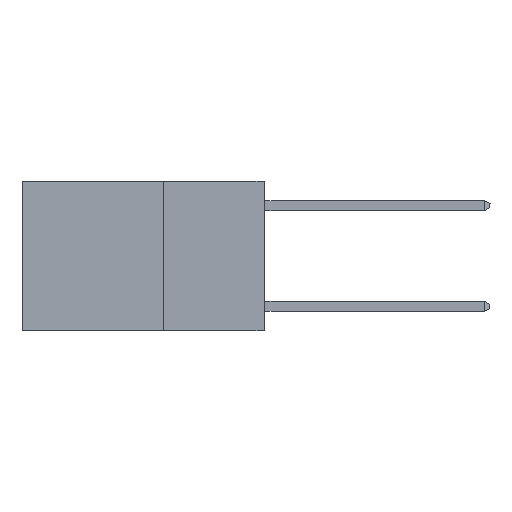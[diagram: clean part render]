
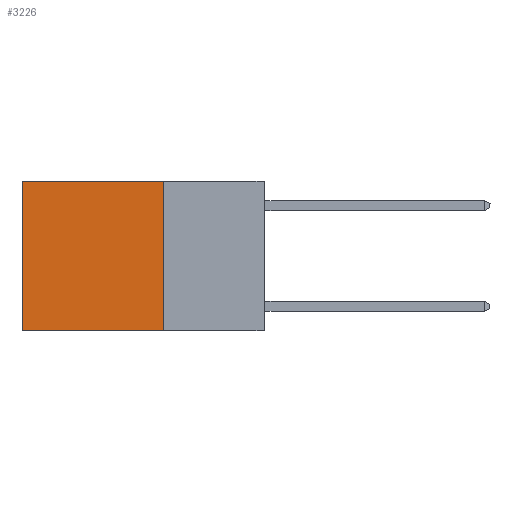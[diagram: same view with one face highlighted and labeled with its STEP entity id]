
A CAD part, left-side view. The second image highlights one B-rep face of the part: STEP entity #3226.
In plain terms, the highlighted planar face has unit normal (-1, 0, 0).
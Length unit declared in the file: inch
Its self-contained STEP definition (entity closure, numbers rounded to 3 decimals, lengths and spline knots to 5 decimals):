
#524 = DIRECTION ( 'NONE',  ( 0., 1., 0. ) ) ;
#903 = AXIS2_PLACEMENT_3D ( 'NONE', #10770, #15862, #12065 ) ;
#1719 = VERTEX_POINT ( 'NONE', #2991 ) ;
#2033 = EDGE_LOOP ( 'NONE', ( #7760, #12344, #16876, #14529 ) ) ;
#2430 = DIRECTION ( 'NONE',  ( 0., 0., -1. ) ) ;
#2991 = CARTESIAN_POINT ( 'NONE',  ( 0.2625, 0.25, 0. ) ) ;
#3226 = ADVANCED_FACE ( 'NONE', ( #10543 ), #19411, .F. ) ;
#3396 = LINE ( 'NONE', #13869, #21032 ) ;
#3861 = VERTEX_POINT ( 'NONE', #16512 ) ;
#4333 = VECTOR ( 'NONE', #524, 39.37008 ) ;
#4805 = EDGE_CURVE ( 'NONE', #1719, #11986, #3396, .T. ) ;
#5864 = CARTESIAN_POINT ( 'NONE',  ( 0.2625, 0.25, 0. ) ) ;
#7760 = ORIENTED_EDGE ( 'NONE', *, *, #21783, .T. ) ;
#8517 = VERTEX_POINT ( 'NONE', #10377 ) ;
#9061 = DIRECTION ( 'NONE',  ( 0., 0., -1. ) ) ;
#9407 = LINE ( 'NONE', #5864, #13550 ) ;
#9446 = EDGE_CURVE ( 'NONE', #3861, #8517, #21908, .T. ) ;
#10377 = CARTESIAN_POINT ( 'NONE',  ( 0.2625, 0.6, -0.37 ) ) ;
#10543 = FACE_OUTER_BOUND ( 'NONE', #2033, .T. ) ;
#10770 = CARTESIAN_POINT ( 'NONE',  ( 0.2625, 0.25, 0. ) ) ;
#11986 = VERTEX_POINT ( 'NONE', #13905 ) ;
#12065 = DIRECTION ( 'NONE',  ( 0., 0., -1. ) ) ;
#12344 = ORIENTED_EDGE ( 'NONE', *, *, #9446, .F. ) ;
#13550 = VECTOR ( 'NONE', #2430, 39.37008 ) ;
#13869 = CARTESIAN_POINT ( 'NONE',  ( 0.2625, 0.25, 0. ) ) ;
#13905 = CARTESIAN_POINT ( 'NONE',  ( 0.2625, 0.6, 0. ) ) ;
#14529 = ORIENTED_EDGE ( 'NONE', *, *, #4805, .T. ) ;
#15862 = DIRECTION ( 'NONE',  ( 1., 0., 0. ) ) ;
#16279 = CARTESIAN_POINT ( 'NONE',  ( 0.2625, 0.25, -0.37 ) ) ;
#16335 = LINE ( 'NONE', #21057, #16472 ) ;
#16472 = VECTOR ( 'NONE', #9061, 39.37008 ) ;
#16512 = CARTESIAN_POINT ( 'NONE',  ( 0.2625, 0.25, -0.37 ) ) ;
#16876 = ORIENTED_EDGE ( 'NONE', *, *, #21836, .F. ) ;
#19363 = DIRECTION ( 'NONE',  ( 0., 1., 0. ) ) ;
#19411 = PLANE ( 'NONE',  #903 ) ;
#21032 = VECTOR ( 'NONE', #19363, 39.37008 ) ;
#21057 = CARTESIAN_POINT ( 'NONE',  ( 0.2625, 0.6, 0. ) ) ;
#21783 = EDGE_CURVE ( 'NONE', #11986, #8517, #16335, .T. ) ;
#21836 = EDGE_CURVE ( 'NONE', #1719, #3861, #9407, .T. ) ;
#21908 = LINE ( 'NONE', #16279, #4333 ) ;
